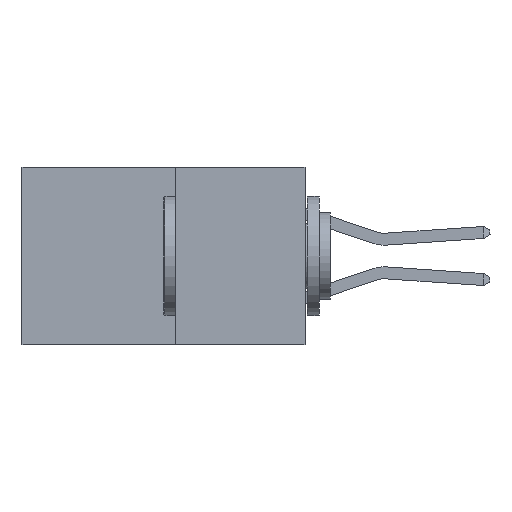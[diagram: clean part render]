
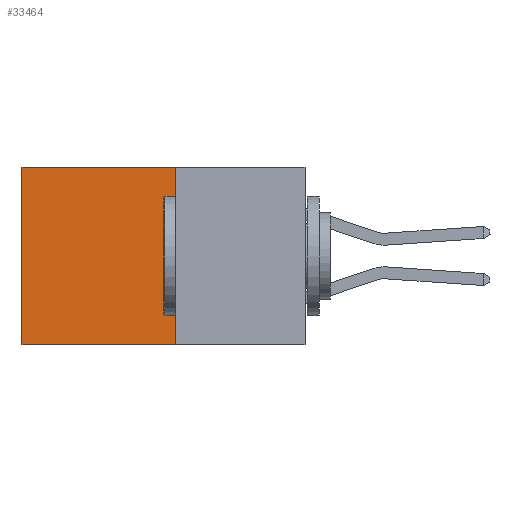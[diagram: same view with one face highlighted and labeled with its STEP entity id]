
A CAD part, left-side view. The second image highlights one B-rep face of the part: STEP entity #33464.
In plain terms, the highlighted planar face has unit normal (-1, 0, 0).
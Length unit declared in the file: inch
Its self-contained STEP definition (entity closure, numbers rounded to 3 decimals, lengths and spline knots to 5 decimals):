
#145 = ORIENTED_EDGE ( 'NONE', *, *, #29503, .T. ) ;
#212 = VECTOR ( 'NONE', #31090, 39.37008 ) ;
#1099 = VERTEX_POINT ( 'NONE', #28293 ) ;
#2599 = VECTOR ( 'NONE', #27724, 39.37008 ) ;
#5046 = EDGE_CURVE ( 'NONE', #6259, #1099, #30226, .T. ) ;
#5208 = ORIENTED_EDGE ( 'NONE', *, *, #26297, .F. ) ;
#6259 = VERTEX_POINT ( 'NONE', #11412 ) ;
#6312 = FACE_OUTER_BOUND ( 'NONE', #33710, .T. ) ;
#6968 = CARTESIAN_POINT ( 'NONE',  ( 0.277, 0.27, -0.37 ) ) ;
#11412 = CARTESIAN_POINT ( 'NONE',  ( 0.277, 0.27, 0. ) ) ;
#11680 = CARTESIAN_POINT ( 'NONE',  ( 0.277, 0.59, -0.37 ) ) ;
#14589 = VERTEX_POINT ( 'NONE', #34790 ) ;
#15312 = DIRECTION ( 'NONE',  ( 0., 0., -1. ) ) ;
#15877 = CARTESIAN_POINT ( 'NONE',  ( 0.277, 0.59, -0.37 ) ) ;
#16097 = LINE ( 'NONE', #6968, #24201 ) ;
#19410 = VECTOR ( 'NONE', #27958, 39.37008 ) ;
#21498 = AXIS2_PLACEMENT_3D ( 'NONE', #34145, #31585, #15312 ) ;
#23764 = ORIENTED_EDGE ( 'NONE', *, *, #5046, .T. ) ;
#24077 = EDGE_CURVE ( 'NONE', #6259, #14589, #16097, .T. ) ;
#24201 = VECTOR ( 'NONE', #26047, 39.37008 ) ;
#24513 = LINE ( 'NONE', #25022, #2599 ) ;
#24608 = ORIENTED_EDGE ( 'NONE', *, *, #24077, .F. ) ;
#25022 = CARTESIAN_POINT ( 'NONE',  ( 0.277, 0.27, -0.37 ) ) ;
#26047 = DIRECTION ( 'NONE',  ( 0., 0., -1. ) ) ;
#26158 = PLANE ( 'NONE',  #21498 ) ;
#26297 = EDGE_CURVE ( 'NONE', #14589, #32238, #24513, .T. ) ;
#27724 = DIRECTION ( 'NONE',  ( 0., 1., 0. ) ) ;
#27958 = DIRECTION ( 'NONE',  ( 0., 0., -1. ) ) ;
#28293 = CARTESIAN_POINT ( 'NONE',  ( 0.277, 0.59, 0. ) ) ;
#29503 = EDGE_CURVE ( 'NONE', #1099, #32238, #34664, .T. ) ;
#30226 = LINE ( 'NONE', #31400, #212 ) ;
#31090 = DIRECTION ( 'NONE',  ( 0., 1., 0. ) ) ;
#31400 = CARTESIAN_POINT ( 'NONE',  ( 0.277, 0.27, 0. ) ) ;
#31585 = DIRECTION ( 'NONE',  ( 1., 0., 0. ) ) ;
#32238 = VERTEX_POINT ( 'NONE', #15877 ) ;
#33464 = ADVANCED_FACE ( 'NONE', ( #6312 ), #26158, .F. ) ;
#33710 = EDGE_LOOP ( 'NONE', ( #145, #5208, #24608, #23764 ) ) ;
#34145 = CARTESIAN_POINT ( 'NONE',  ( 0.277, 0.27, -0.37 ) ) ;
#34664 = LINE ( 'NONE', #11680, #19410 ) ;
#34790 = CARTESIAN_POINT ( 'NONE',  ( 0.277, 0.27, -0.37 ) ) ;
